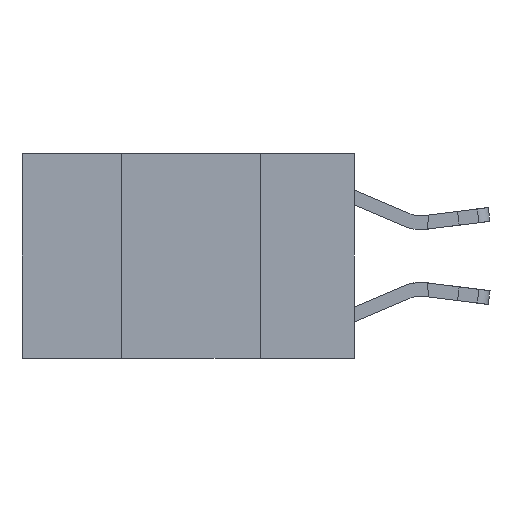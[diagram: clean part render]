
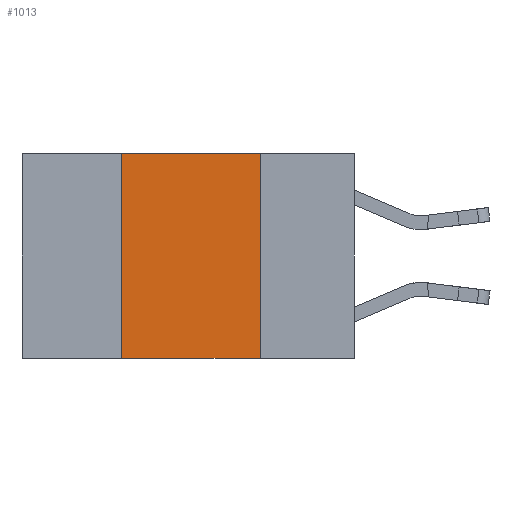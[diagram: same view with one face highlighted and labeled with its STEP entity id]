
A CAD part, left-side view. The second image highlights one B-rep face of the part: STEP entity #1013.
In plain terms, the highlighted planar face has unit normal (-1, 0, 0).
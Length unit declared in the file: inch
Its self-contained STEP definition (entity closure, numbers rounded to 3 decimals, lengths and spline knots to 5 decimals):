
#75 = CARTESIAN_POINT ( 'NONE',  ( 0., 0.6, 0. ) ) ;
#184 = VECTOR ( 'NONE', #10425, 39.37008 ) ;
#1013 = ADVANCED_FACE ( 'NONE', ( #1692 ), #9992, .F. ) ;
#1502 = EDGE_CURVE ( 'NONE', #5004, #13977, #14470, .T. ) ;
#1692 = FACE_OUTER_BOUND ( 'NONE', #13897, .T. ) ;
#2157 = DIRECTION ( 'NONE',  ( 0., 0., -1. ) ) ;
#2207 = CARTESIAN_POINT ( 'NONE',  ( 0., 0.6, -0.37 ) ) ;
#3121 = VERTEX_POINT ( 'NONE', #5542 ) ;
#3475 = ORIENTED_EDGE ( 'NONE', *, *, #5780, .F. ) ;
#3777 = VERTEX_POINT ( 'NONE', #10236 ) ;
#5004 = VERTEX_POINT ( 'NONE', #14229 ) ;
#5542 = CARTESIAN_POINT ( 'NONE',  ( 0., 0.42, 0. ) ) ;
#5556 = EDGE_CURVE ( 'NONE', #5004, #3121, #10754, .T. ) ;
#5780 = EDGE_CURVE ( 'NONE', #3777, #13977, #14606, .T. ) ;
#7277 = ORIENTED_EDGE ( 'NONE', *, *, #12302, .F. ) ;
#7580 = CARTESIAN_POINT ( 'NONE',  ( 0., 0.6, 0. ) ) ;
#8012 = DIRECTION ( 'NONE',  ( 0., 0., 1. ) ) ;
#8271 = AXIS2_PLACEMENT_3D ( 'NONE', #75, #16616, #11163 ) ;
#9992 = PLANE ( 'NONE',  #8271 ) ;
#10236 = CARTESIAN_POINT ( 'NONE',  ( 0., 0.17, 0. ) ) ;
#10425 = DIRECTION ( 'NONE',  ( 0., -1., 0. ) ) ;
#10490 = CARTESIAN_POINT ( 'NONE',  ( 0., 0.42, 0. ) ) ;
#10754 = LINE ( 'NONE', #10490, #13356 ) ;
#11163 = DIRECTION ( 'NONE',  ( 0., 0., -1. ) ) ;
#11546 = DIRECTION ( 'NONE',  ( 0., -1., 0. ) ) ;
#11921 = LINE ( 'NONE', #7580, #184 ) ;
#12302 = EDGE_CURVE ( 'NONE', #3121, #3777, #11921, .T. ) ;
#13235 = VECTOR ( 'NONE', #2157, 39.37008 ) ;
#13356 = VECTOR ( 'NONE', #8012, 39.37008 ) ;
#13897 = EDGE_LOOP ( 'NONE', ( #3475, #7277, #15405, #17467 ) ) ;
#13977 = VERTEX_POINT ( 'NONE', #17480 ) ;
#14229 = CARTESIAN_POINT ( 'NONE',  ( 0., 0.42, -0.37 ) ) ;
#14470 = LINE ( 'NONE', #2207, #16652 ) ;
#14606 = LINE ( 'NONE', #15874, #13235 ) ;
#15405 = ORIENTED_EDGE ( 'NONE', *, *, #5556, .F. ) ;
#15874 = CARTESIAN_POINT ( 'NONE',  ( 0., 0.17, 0. ) ) ;
#16616 = DIRECTION ( 'NONE',  ( 1., 0., 0. ) ) ;
#16652 = VECTOR ( 'NONE', #11546, 39.37008 ) ;
#17467 = ORIENTED_EDGE ( 'NONE', *, *, #1502, .T. ) ;
#17480 = CARTESIAN_POINT ( 'NONE',  ( 0., 0.17, -0.37 ) ) ;
